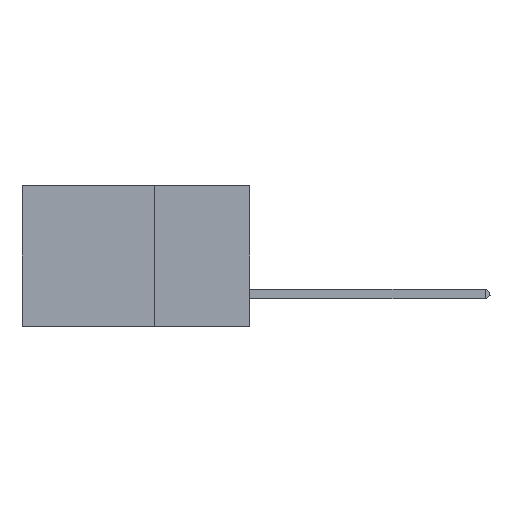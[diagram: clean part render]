
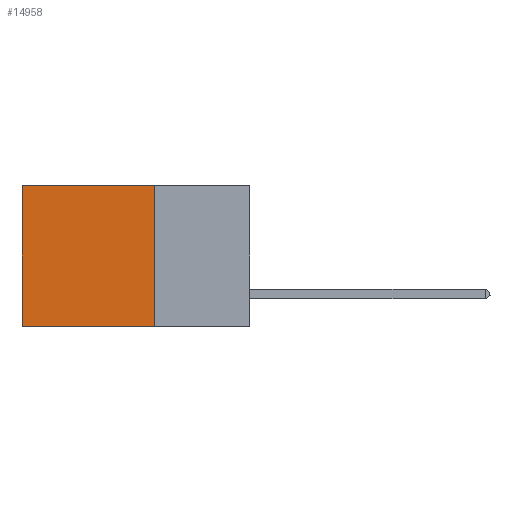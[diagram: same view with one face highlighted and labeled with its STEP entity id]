
A CAD part, left-side view. The second image highlights one B-rep face of the part: STEP entity #14958.
In plain terms, the highlighted planar face has unit normal (-1, 0, 0).
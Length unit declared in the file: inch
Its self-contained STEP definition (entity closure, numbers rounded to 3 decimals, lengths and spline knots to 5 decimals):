
#268 = CARTESIAN_POINT ( 'NONE',  ( 0.2875, 0.25, 0. ) ) ;
#2288 = LINE ( 'NONE', #10848, #15441 ) ;
#3252 = AXIS2_PLACEMENT_3D ( 'NONE', #268, #13088, #6878 ) ;
#3253 = EDGE_CURVE ( 'NONE', #22595, #20985, #26672, .T. ) ;
#3810 = EDGE_CURVE ( 'NONE', #22595, #8777, #2288, .T. ) ;
#4514 = ORIENTED_EDGE ( 'NONE', *, *, #12098, .T. ) ;
#4729 = CARTESIAN_POINT ( 'NONE',  ( 0.2875, 0.6, -0.37 ) ) ;
#5371 = VECTOR ( 'NONE', #16072, 39.37008 ) ;
#6534 = DIRECTION ( 'NONE',  ( 0., 0., -1. ) ) ;
#6878 = DIRECTION ( 'NONE',  ( 0., 0., -1. ) ) ;
#6918 = EDGE_CURVE ( 'NONE', #8777, #12245, #18551, .T. ) ;
#8777 = VERTEX_POINT ( 'NONE', #14289 ) ;
#9884 = EDGE_LOOP ( 'NONE', ( #4514, #11759, #26611, #15644 ) ) ;
#10690 = DIRECTION ( 'NONE',  ( 0., 1., 0. ) ) ;
#10848 = CARTESIAN_POINT ( 'NONE',  ( 0.2875, 0.25, 0. ) ) ;
#11076 = CARTESIAN_POINT ( 'NONE',  ( 0.2875, 0.6, 0. ) ) ;
#11444 = DIRECTION ( 'NONE',  ( 0., 0., -1. ) ) ;
#11759 = ORIENTED_EDGE ( 'NONE', *, *, #6918, .F. ) ;
#12098 = EDGE_CURVE ( 'NONE', #20985, #12245, #14283, .T. ) ;
#12245 = VERTEX_POINT ( 'NONE', #4729 ) ;
#13088 = DIRECTION ( 'NONE',  ( 1., 0., 0. ) ) ;
#14283 = LINE ( 'NONE', #11076, #15960 ) ;
#14289 = CARTESIAN_POINT ( 'NONE',  ( 0.2875, 0.25, -0.37 ) ) ;
#14958 = ADVANCED_FACE ( 'NONE', ( #15829 ), #25451, .F. ) ;
#15441 = VECTOR ( 'NONE', #6534, 39.37008 ) ;
#15644 = ORIENTED_EDGE ( 'NONE', *, *, #3253, .T. ) ;
#15829 = FACE_OUTER_BOUND ( 'NONE', #9884, .T. ) ;
#15960 = VECTOR ( 'NONE', #11444, 39.37008 ) ;
#16030 = CARTESIAN_POINT ( 'NONE',  ( 0.2875, 0.25, 0. ) ) ;
#16072 = DIRECTION ( 'NONE',  ( 0., 1., 0. ) ) ;
#17081 = CARTESIAN_POINT ( 'NONE',  ( 0.2875, 0.25, 0. ) ) ;
#18031 = CARTESIAN_POINT ( 'NONE',  ( 0.2875, 0.25, -0.37 ) ) ;
#18551 = LINE ( 'NONE', #18031, #5371 ) ;
#20985 = VERTEX_POINT ( 'NONE', #21676 ) ;
#21676 = CARTESIAN_POINT ( 'NONE',  ( 0.2875, 0.6, 0. ) ) ;
#22595 = VERTEX_POINT ( 'NONE', #16030 ) ;
#25451 = PLANE ( 'NONE',  #3252 ) ;
#25667 = VECTOR ( 'NONE', #10690, 39.37008 ) ;
#26611 = ORIENTED_EDGE ( 'NONE', *, *, #3810, .F. ) ;
#26672 = LINE ( 'NONE', #17081, #25667 ) ;
